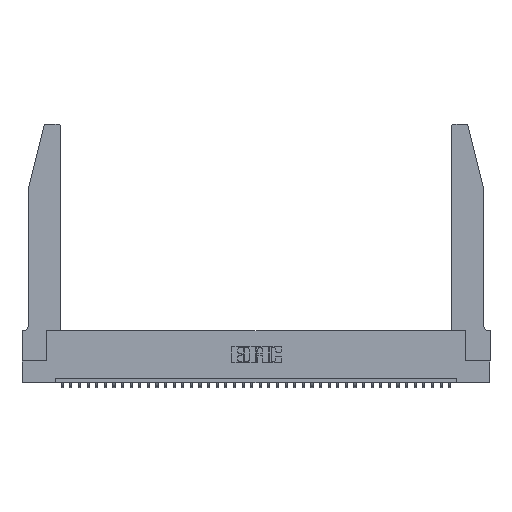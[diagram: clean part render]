
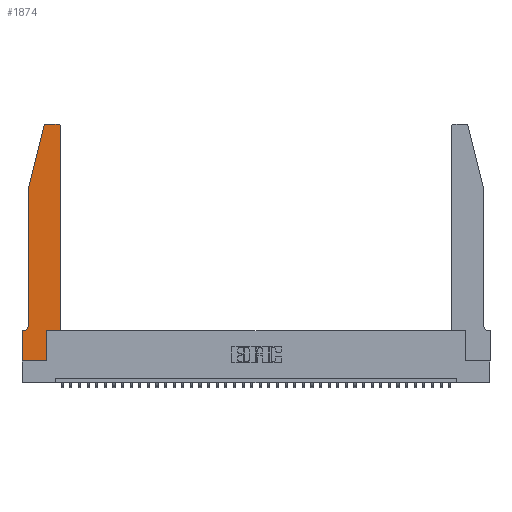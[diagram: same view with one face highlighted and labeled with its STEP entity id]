
A CAD part, top view. The second image highlights one B-rep face of the part: STEP entity #1874.
In plain terms, the highlighted planar face has unit normal (0, 0, 1).
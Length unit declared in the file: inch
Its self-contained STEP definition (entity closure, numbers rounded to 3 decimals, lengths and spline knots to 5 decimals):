
#154 = CARTESIAN_POINT ( 'NONE',  ( 0., 0., 0.37 ) ) ;
#274 = EDGE_CURVE ( 'NONE', #6836, #12255, #30724, .T. ) ;
#407 = CARTESIAN_POINT ( 'NONE',  ( 0.0755, 0.42, 0.37 ) ) ;
#702 = EDGE_CURVE ( 'NONE', #17300, #12318, #35859, .T. ) ;
#1176 = CARTESIAN_POINT ( 'NONE',  ( 0., 0.35, 0.37 ) ) ;
#1217 = ORIENTED_EDGE ( 'NONE', *, *, #274, .T. ) ;
#1366 = AXIS2_PLACEMENT_3D ( 'NONE', #10994, #25725, #5241 ) ;
#1496 = VECTOR ( 'NONE', #4840, 39.37008 ) ;
#1874 = ADVANCED_FACE ( 'NONE', ( #28675 ), #25859, .T. ) ;
#2886 = ORIENTED_EDGE ( 'NONE', *, *, #6469, .T. ) ;
#3026 = EDGE_CURVE ( 'NONE', #32942, #6265, #37034, .T. ) ;
#3745 = LINE ( 'NONE', #27461, #17863 ) ;
#4222 = CARTESIAN_POINT ( 'NONE',  ( 0.0755, 2., 0.37 ) ) ;
#4631 = AXIS2_PLACEMENT_3D ( 'NONE', #37014, #9951, #18913 ) ;
#4840 = DIRECTION ( 'NONE',  ( -1., 0., 0. ) ) ;
#4888 = VECTOR ( 'NONE', #31360, 39.37008 ) ;
#5241 = DIRECTION ( 'NONE',  ( 1., 0., 0. ) ) ;
#5841 = DIRECTION ( 'NONE',  ( -1., 0., 0. ) ) ;
#5968 = DIRECTION ( 'NONE',  ( 0., 0., -1. ) ) ;
#6083 = CARTESIAN_POINT ( 'NONE',  ( 0.25487, 2.72718, 0.37 ) ) ;
#6265 = VERTEX_POINT ( 'NONE', #17078 ) ;
#6319 = DIRECTION ( 'NONE',  ( 1., 0., 0. ) ) ;
#6469 = EDGE_CURVE ( 'NONE', #12318, #22354, #34785, .T. ) ;
#6836 = VERTEX_POINT ( 'NONE', #30839 ) ;
#7317 = LINE ( 'NONE', #38607, #28474 ) ;
#7622 = ORIENTED_EDGE ( 'NONE', *, *, #35049, .T. ) ;
#7838 = LINE ( 'NONE', #12635, #22420 ) ;
#8526 = CARTESIAN_POINT ( 'NONE',  ( 0.2865, 0.35, 0.37 ) ) ;
#8864 = VECTOR ( 'NONE', #21847, 39.37008 ) ;
#8936 = VECTOR ( 'NONE', #29541, 39.37008 ) ;
#9512 = ORIENTED_EDGE ( 'NONE', *, *, #12668, .T. ) ;
#9951 = DIRECTION ( 'NONE',  ( 0., 0., 1. ) ) ;
#9985 = ORIENTED_EDGE ( 'NONE', *, *, #25313, .T. ) ;
#10071 = CARTESIAN_POINT ( 'NONE',  ( 0.2605, 2.75, 0.37 ) ) ;
#10144 = ORIENTED_EDGE ( 'NONE', *, *, #22630, .T. ) ;
#10598 = ORIENTED_EDGE ( 'NONE', *, *, #702, .T. ) ;
#10994 = CARTESIAN_POINT ( 'NONE',  ( 0., 0.35, 0.37 ) ) ;
#11519 = LINE ( 'NONE', #22549, #20020 ) ;
#12255 = VERTEX_POINT ( 'NONE', #25696 ) ;
#12318 = VERTEX_POINT ( 'NONE', #14289 ) ;
#12390 = ORIENTED_EDGE ( 'NONE', *, *, #35983, .T. ) ;
#12635 = CARTESIAN_POINT ( 'NONE',  ( 0., 0., 0.37 ) ) ;
#12668 = EDGE_CURVE ( 'NONE', #6265, #17302, #7317, .T. ) ;
#13131 = DIRECTION ( 'NONE',  ( 1., 0., 0. ) ) ;
#13218 = DIRECTION ( 'NONE',  ( 0., 1., 0. ) ) ;
#14235 = EDGE_CURVE ( 'NONE', #36996, #32942, #28825, .T. ) ;
#14289 = CARTESIAN_POINT ( 'NONE',  ( 0.2865, 0., 0.37 ) ) ;
#14681 = VERTEX_POINT ( 'NONE', #21775 ) ;
#14767 = CARTESIAN_POINT ( 'NONE',  ( 0.0055, 0.42, 0.37 ) ) ;
#16784 = DIRECTION ( 'NONE',  ( 0., -1., 0. ) ) ;
#17078 = CARTESIAN_POINT ( 'NONE',  ( 0.0755, 2., 0.37 ) ) ;
#17300 = VERTEX_POINT ( 'NONE', #154 ) ;
#17302 = VERTEX_POINT ( 'NONE', #407 ) ;
#17863 = VECTOR ( 'NONE', #6319, 39.37008 ) ;
#17913 = ORIENTED_EDGE ( 'NONE', *, *, #34016, .T. ) ;
#18913 = DIRECTION ( 'NONE',  ( 1., 0., 0. ) ) ;
#19685 = CARTESIAN_POINT ( 'NONE',  ( 0.0755, 0.35, 0.37 ) ) ;
#19888 = CARTESIAN_POINT ( 'NONE',  ( 0.2865, 0.35, 0.37 ) ) ;
#20020 = VECTOR ( 'NONE', #13218, 39.37008 ) ;
#20220 = CARTESIAN_POINT ( 'NONE',  ( 0.4205, 2.72, 0.37 ) ) ;
#20502 = VERTEX_POINT ( 'NONE', #34800 ) ;
#20815 = LINE ( 'NONE', #19685, #1496 ) ;
#21775 = CARTESIAN_POINT ( 'NONE',  ( 0.4505, 0.35, 0.37 ) ) ;
#21847 = DIRECTION ( 'NONE',  ( -0.239, -0.971, 0. ) ) ;
#22354 = VERTEX_POINT ( 'NONE', #19888 ) ;
#22420 = VECTOR ( 'NONE', #33922, 39.37008 ) ;
#22549 = CARTESIAN_POINT ( 'NONE',  ( 0.4505, 0.35, 0.37 ) ) ;
#22630 = EDGE_CURVE ( 'NONE', #17302, #20502, #27949, .T. ) ;
#23039 = ORIENTED_EDGE ( 'NONE', *, *, #14235, .T. ) ;
#25313 = EDGE_CURVE ( 'NONE', #12255, #36996, #34515, .T. ) ;
#25696 = CARTESIAN_POINT ( 'NONE',  ( 0.4205, 2.75, 0.37 ) ) ;
#25725 = DIRECTION ( 'NONE',  ( 0., 0., 1. ) ) ;
#25859 = PLANE ( 'NONE',  #1366 ) ;
#27074 = EDGE_CURVE ( 'NONE', #20502, #37699, #20815, .T. ) ;
#27461 = CARTESIAN_POINT ( 'NONE',  ( 0.4505, 0.35, 0.37 ) ) ;
#27917 = ORIENTED_EDGE ( 'NONE', *, *, #27074, .T. ) ;
#27949 = CIRCLE ( 'NONE', #28736, 0.07 ) ;
#28335 = VECTOR ( 'NONE', #13131, 39.37008 ) ;
#28474 = VECTOR ( 'NONE', #16784, 39.37008 ) ;
#28675 = FACE_OUTER_BOUND ( 'NONE', #33803, .T. ) ;
#28736 = AXIS2_PLACEMENT_3D ( 'NONE', #14767, #5968, #5841 ) ;
#28825 = CIRCLE ( 'NONE', #4631, 0.03 ) ;
#29541 = DIRECTION ( 'NONE',  ( 0., 1., 0. ) ) ;
#30561 = AXIS2_PLACEMENT_3D ( 'NONE', #20220, #38588, #32313 ) ;
#30724 = CIRCLE ( 'NONE', #30561, 0.03 ) ;
#30839 = CARTESIAN_POINT ( 'NONE',  ( 0.4505, 2.72, 0.37 ) ) ;
#31360 = DIRECTION ( 'NONE',  ( -1., 0., 0. ) ) ;
#32313 = DIRECTION ( 'NONE',  ( 1., 0., 0. ) ) ;
#32942 = VERTEX_POINT ( 'NONE', #6083 ) ;
#32976 = ORIENTED_EDGE ( 'NONE', *, *, #3026, .T. ) ;
#33053 = CARTESIAN_POINT ( 'NONE',  ( 0.284, 2.75, 0.37 ) ) ;
#33803 = EDGE_LOOP ( 'NONE', ( #9985, #23039, #32976, #9512, #10144, #27917, #7622, #10598, #2886, #17913, #12390, #1217 ) ) ;
#33922 = DIRECTION ( 'NONE',  ( 0., -1., 0. ) ) ;
#34016 = EDGE_CURVE ( 'NONE', #22354, #14681, #3745, .T. ) ;
#34427 = CARTESIAN_POINT ( 'NONE',  ( 0., 0., 0.37 ) ) ;
#34515 = LINE ( 'NONE', #10071, #4888 ) ;
#34785 = LINE ( 'NONE', #8526, #8936 ) ;
#34800 = CARTESIAN_POINT ( 'NONE',  ( 0.0055, 0.35, 0.37 ) ) ;
#35049 = EDGE_CURVE ( 'NONE', #37699, #17300, #7838, .T. ) ;
#35859 = LINE ( 'NONE', #34427, #28335 ) ;
#35983 = EDGE_CURVE ( 'NONE', #14681, #6836, #11519, .T. ) ;
#36996 = VERTEX_POINT ( 'NONE', #33053 ) ;
#37014 = CARTESIAN_POINT ( 'NONE',  ( 0.284, 2.72, 0.37 ) ) ;
#37034 = LINE ( 'NONE', #4222, #8864 ) ;
#37699 = VERTEX_POINT ( 'NONE', #1176 ) ;
#38588 = DIRECTION ( 'NONE',  ( 0., 0., 1. ) ) ;
#38607 = CARTESIAN_POINT ( 'NONE',  ( 0.0755, 2., 0.37 ) ) ;
